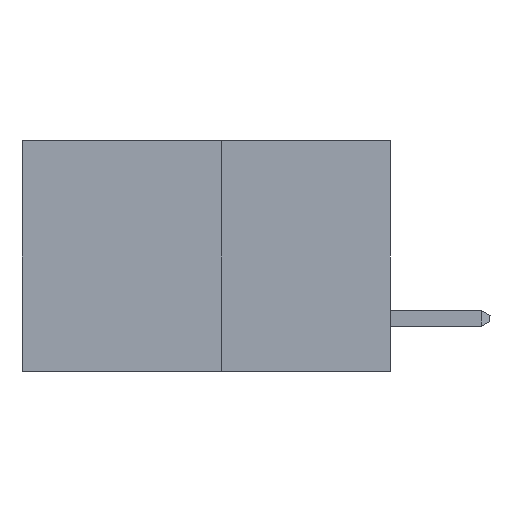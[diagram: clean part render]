
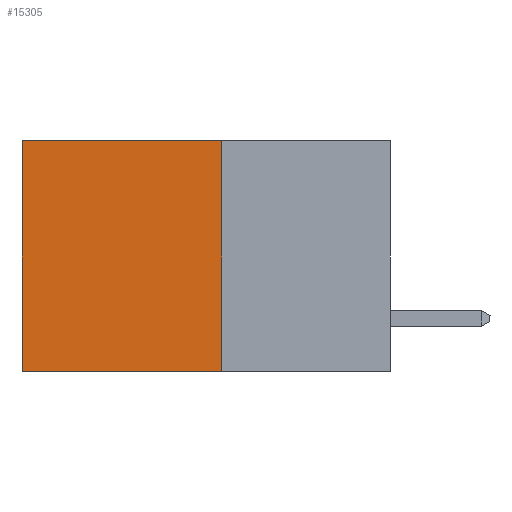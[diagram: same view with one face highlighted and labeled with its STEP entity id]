
A CAD part, left-side view. The second image highlights one B-rep face of the part: STEP entity #15305.
In plain terms, the highlighted planar face has unit normal (-1, 0, 0).
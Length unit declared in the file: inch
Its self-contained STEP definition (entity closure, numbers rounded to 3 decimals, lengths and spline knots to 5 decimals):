
#575 = LINE ( 'NONE', #6508, #13381 ) ;
#670 = CARTESIAN_POINT ( 'NONE',  ( 0.277, 0.27, 0. ) ) ;
#911 = DIRECTION ( 'NONE',  ( 0., 0., -1. ) ) ;
#1229 = DIRECTION ( 'NONE',  ( 0., 0., -1. ) ) ;
#1580 = DIRECTION ( 'NONE',  ( 0., 1., 0. ) ) ;
#2137 = LINE ( 'NONE', #12424, #14184 ) ;
#2455 = VERTEX_POINT ( 'NONE', #9380 ) ;
#2458 = EDGE_CURVE ( 'NONE', #11623, #7678, #14326, .T. ) ;
#2603 = ORIENTED_EDGE ( 'NONE', *, *, #2458, .F. ) ;
#3607 = ORIENTED_EDGE ( 'NONE', *, *, #11433, .T. ) ;
#4314 = CARTESIAN_POINT ( 'NONE',  ( 0.277, 0.27, -0.37 ) ) ;
#4765 = CARTESIAN_POINT ( 'NONE',  ( 0.277, 0.27, -0.37 ) ) ;
#5245 = VECTOR ( 'NONE', #14427, 39.37008 ) ;
#5629 = DIRECTION ( 'NONE',  ( 0., 0., -1. ) ) ;
#6088 = VERTEX_POINT ( 'NONE', #6222 ) ;
#6222 = CARTESIAN_POINT ( 'NONE',  ( 0.277, 0.59, -0.37 ) ) ;
#6508 = CARTESIAN_POINT ( 'NONE',  ( 0.277, 0.27, 0. ) ) ;
#6830 = EDGE_CURVE ( 'NONE', #7678, #6088, #15177, .T. ) ;
#7091 = EDGE_CURVE ( 'NONE', #2455, #6088, #2137, .T. ) ;
#7678 = VERTEX_POINT ( 'NONE', #4765 ) ;
#7917 = ORIENTED_EDGE ( 'NONE', *, *, #6830, .F. ) ;
#9380 = CARTESIAN_POINT ( 'NONE',  ( 0.277, 0.59, 0. ) ) ;
#11020 = VECTOR ( 'NONE', #911, 39.37008 ) ;
#11433 = EDGE_CURVE ( 'NONE', #11623, #2455, #575, .T. ) ;
#11623 = VERTEX_POINT ( 'NONE', #670 ) ;
#11814 = PLANE ( 'NONE',  #13864 ) ;
#11915 = CARTESIAN_POINT ( 'NONE',  ( 0.277, 0.27, -0.37 ) ) ;
#12424 = CARTESIAN_POINT ( 'NONE',  ( 0.277, 0.59, -0.37 ) ) ;
#13065 = DIRECTION ( 'NONE',  ( 1., 0., 0. ) ) ;
#13381 = VECTOR ( 'NONE', #1580, 39.37008 ) ;
#13864 = AXIS2_PLACEMENT_3D ( 'NONE', #4314, #13065, #5629 ) ;
#14184 = VECTOR ( 'NONE', #1229, 39.37008 ) ;
#14325 = EDGE_LOOP ( 'NONE', ( #15201, #7917, #2603, #3607 ) ) ;
#14326 = LINE ( 'NONE', #11915, #11020 ) ;
#14427 = DIRECTION ( 'NONE',  ( 0., 1., 0. ) ) ;
#15177 = LINE ( 'NONE', #15625, #5245 ) ;
#15201 = ORIENTED_EDGE ( 'NONE', *, *, #7091, .T. ) ;
#15305 = ADVANCED_FACE ( 'NONE', ( #15326 ), #11814, .F. ) ;
#15326 = FACE_OUTER_BOUND ( 'NONE', #14325, .T. ) ;
#15625 = CARTESIAN_POINT ( 'NONE',  ( 0.277, 0.27, -0.37 ) ) ;
